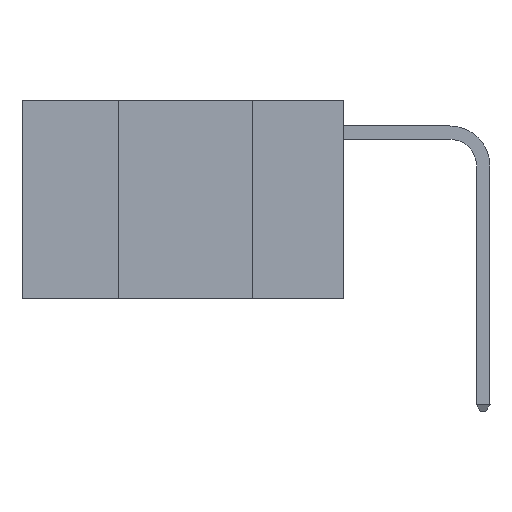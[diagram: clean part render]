
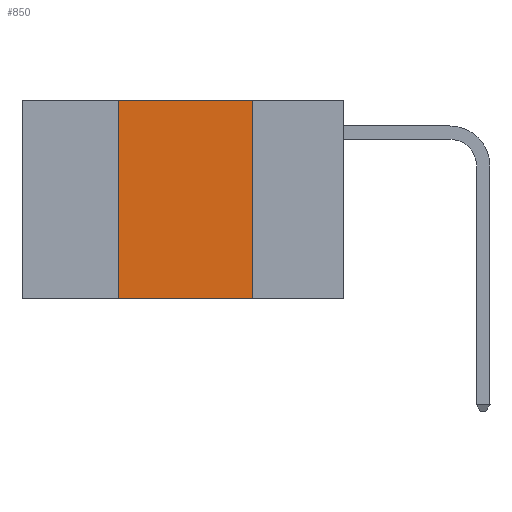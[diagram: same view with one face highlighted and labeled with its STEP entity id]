
A CAD part, left-side view. The second image highlights one B-rep face of the part: STEP entity #850.
In plain terms, the highlighted planar face has unit normal (-1, 0, 0).
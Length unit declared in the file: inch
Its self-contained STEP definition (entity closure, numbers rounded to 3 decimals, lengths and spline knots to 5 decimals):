
#850 = ADVANCED_FACE ( 'NONE', ( #5739 ), #6249, .F. ) ;
#1454 = VERTEX_POINT ( 'NONE', #4783 ) ;
#2126 = EDGE_CURVE ( 'NONE', #3927, #6671, #9452, .T. ) ;
#2570 = LINE ( 'NONE', #10687, #5350 ) ;
#3087 = EDGE_CURVE ( 'NONE', #7137, #6671, #2570, .T. ) ;
#3334 = DIRECTION ( 'NONE',  ( 0., 0., -1. ) ) ;
#3927 = VERTEX_POINT ( 'NONE', #5691 ) ;
#4204 = CARTESIAN_POINT ( 'NONE',  ( 0., 0.6, 0. ) ) ;
#4783 = CARTESIAN_POINT ( 'NONE',  ( 0., 0.42, 0. ) ) ;
#5089 = CARTESIAN_POINT ( 'NONE',  ( 0., 0.6, 0. ) ) ;
#5266 = DIRECTION ( 'NONE',  ( 1., 0., 0. ) ) ;
#5274 = EDGE_CURVE ( 'NONE', #7137, #1454, #11515, .T. ) ;
#5350 = VECTOR ( 'NONE', #11318, 39.37008 ) ;
#5691 = CARTESIAN_POINT ( 'NONE',  ( 0., 0.17, 0. ) ) ;
#5739 = FACE_OUTER_BOUND ( 'NONE', #10396, .T. ) ;
#6249 = PLANE ( 'NONE',  #11710 ) ;
#6671 = VERTEX_POINT ( 'NONE', #9694 ) ;
#7137 = VERTEX_POINT ( 'NONE', #12768 ) ;
#7141 = CARTESIAN_POINT ( 'NONE',  ( 0., 0.42, 0. ) ) ;
#7256 = DIRECTION ( 'NONE',  ( 0., 0., 1. ) ) ;
#7507 = EDGE_CURVE ( 'NONE', #1454, #3927, #12756, .T. ) ;
#7723 = CARTESIAN_POINT ( 'NONE',  ( 0., 0.17, 0. ) ) ;
#7754 = DIRECTION ( 'NONE',  ( 0., 0., -1. ) ) ;
#7868 = VECTOR ( 'NONE', #11299, 39.37008 ) ;
#9452 = LINE ( 'NONE', #7723, #12241 ) ;
#9694 = CARTESIAN_POINT ( 'NONE',  ( 0., 0.17, -0.37 ) ) ;
#10396 = EDGE_LOOP ( 'NONE', ( #11093, #12577, #12542, #11931 ) ) ;
#10687 = CARTESIAN_POINT ( 'NONE',  ( 0., 0.6, -0.37 ) ) ;
#11093 = ORIENTED_EDGE ( 'NONE', *, *, #2126, .F. ) ;
#11184 = VECTOR ( 'NONE', #7256, 39.37008 ) ;
#11299 = DIRECTION ( 'NONE',  ( 0., -1., 0. ) ) ;
#11318 = DIRECTION ( 'NONE',  ( 0., -1., 0. ) ) ;
#11515 = LINE ( 'NONE', #7141, #11184 ) ;
#11710 = AXIS2_PLACEMENT_3D ( 'NONE', #4204, #5266, #3334 ) ;
#11931 = ORIENTED_EDGE ( 'NONE', *, *, #3087, .T. ) ;
#12241 = VECTOR ( 'NONE', #7754, 39.37008 ) ;
#12542 = ORIENTED_EDGE ( 'NONE', *, *, #5274, .F. ) ;
#12577 = ORIENTED_EDGE ( 'NONE', *, *, #7507, .F. ) ;
#12756 = LINE ( 'NONE', #5089, #7868 ) ;
#12768 = CARTESIAN_POINT ( 'NONE',  ( 0., 0.42, -0.37 ) ) ;
